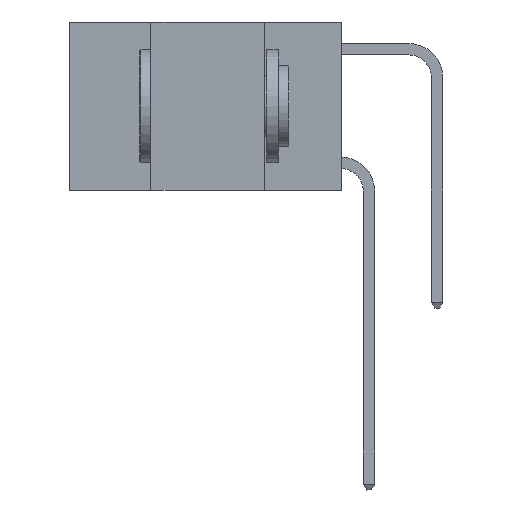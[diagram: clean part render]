
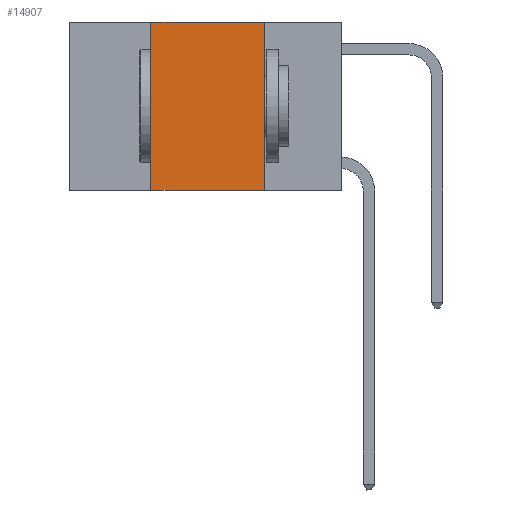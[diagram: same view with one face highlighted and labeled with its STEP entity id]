
A CAD part, left-side view. The second image highlights one B-rep face of the part: STEP entity #14907.
In plain terms, the highlighted planar face has unit normal (-1, 0, 0).
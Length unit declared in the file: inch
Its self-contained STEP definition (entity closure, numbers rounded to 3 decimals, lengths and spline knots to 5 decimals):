
#240 = CARTESIAN_POINT ( 'NONE',  ( 0., 0.17, -0.37 ) ) ;
#742 = LINE ( 'NONE', #6524, #6552 ) ;
#1551 = CARTESIAN_POINT ( 'NONE',  ( 0., 0.42, 0. ) ) ;
#2054 = CARTESIAN_POINT ( 'NONE',  ( 0., 0.42, 0. ) ) ;
#2188 = EDGE_CURVE ( 'NONE', #4576, #3366, #742, .T. ) ;
#3366 = VERTEX_POINT ( 'NONE', #240 ) ;
#3841 = ORIENTED_EDGE ( 'NONE', *, *, #14883, .F. ) ;
#4050 = DIRECTION ( 'NONE',  ( 0., 0., -1. ) ) ;
#4499 = VECTOR ( 'NONE', #13038, 39.37008 ) ;
#4576 = VERTEX_POINT ( 'NONE', #10801 ) ;
#5676 = FACE_OUTER_BOUND ( 'NONE', #16192, .T. ) ;
#6524 = CARTESIAN_POINT ( 'NONE',  ( 0., 0.6, -0.37 ) ) ;
#6552 = VECTOR ( 'NONE', #8212, 39.37008 ) ;
#7016 = CARTESIAN_POINT ( 'NONE',  ( 0., 0.17, 0. ) ) ;
#7107 = ORIENTED_EDGE ( 'NONE', *, *, #2188, .T. ) ;
#7113 = VERTEX_POINT ( 'NONE', #13865 ) ;
#8212 = DIRECTION ( 'NONE',  ( 0., -1., 0. ) ) ;
#9928 = VERTEX_POINT ( 'NONE', #1551 ) ;
#10774 = LINE ( 'NONE', #7016, #13545 ) ;
#10801 = CARTESIAN_POINT ( 'NONE',  ( 0., 0.42, -0.37 ) ) ;
#11614 = DIRECTION ( 'NONE',  ( 1., 0., 0. ) ) ;
#12329 = ORIENTED_EDGE ( 'NONE', *, *, #15980, .F. ) ;
#13038 = DIRECTION ( 'NONE',  ( 0., 0., 1. ) ) ;
#13220 = PLANE ( 'NONE',  #20512 ) ;
#13545 = VECTOR ( 'NONE', #18286, 39.37008 ) ;
#13865 = CARTESIAN_POINT ( 'NONE',  ( 0., 0.17, 0. ) ) ;
#14468 = DIRECTION ( 'NONE',  ( 0., -1., 0. ) ) ;
#14713 = LINE ( 'NONE', #24181, #20894 ) ;
#14883 = EDGE_CURVE ( 'NONE', #9928, #7113, #14713, .T. ) ;
#14907 = ADVANCED_FACE ( 'NONE', ( #5676 ), #13220, .F. ) ;
#15980 = EDGE_CURVE ( 'NONE', #4576, #9928, #20581, .T. ) ;
#16192 = EDGE_LOOP ( 'NONE', ( #20075, #3841, #12329, #7107 ) ) ;
#18286 = DIRECTION ( 'NONE',  ( 0., 0., -1. ) ) ;
#18552 = EDGE_CURVE ( 'NONE', #7113, #3366, #10774, .T. ) ;
#20075 = ORIENTED_EDGE ( 'NONE', *, *, #18552, .F. ) ;
#20512 = AXIS2_PLACEMENT_3D ( 'NONE', #20763, #11614, #4050 ) ;
#20581 = LINE ( 'NONE', #2054, #4499 ) ;
#20763 = CARTESIAN_POINT ( 'NONE',  ( 0., 0.6, 0. ) ) ;
#20894 = VECTOR ( 'NONE', #14468, 39.37008 ) ;
#24181 = CARTESIAN_POINT ( 'NONE',  ( 0., 0.6, 0. ) ) ;
